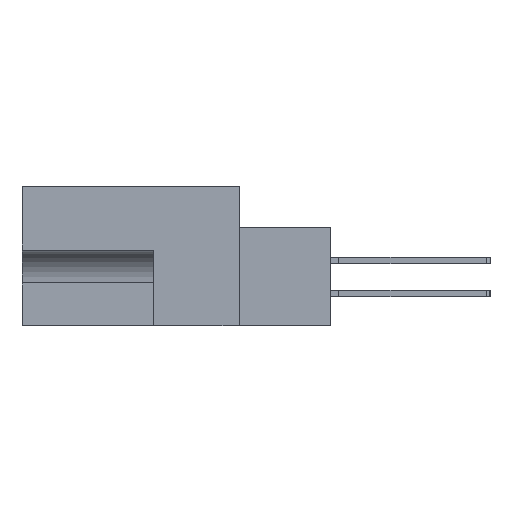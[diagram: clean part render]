
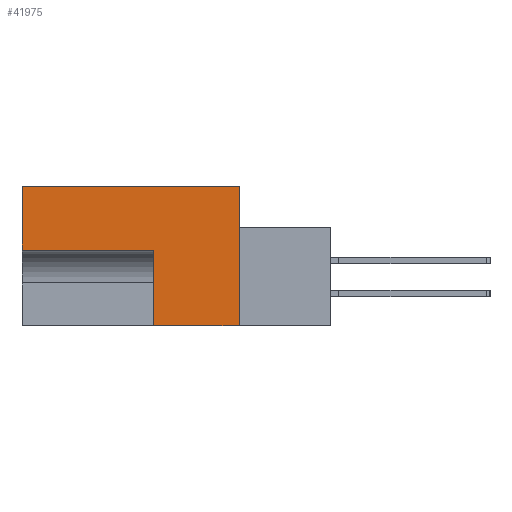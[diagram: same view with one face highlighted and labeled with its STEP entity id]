
A CAD part, left-side view. The second image highlights one B-rep face of the part: STEP entity #41975.
In plain terms, the highlighted planar face has unit normal (-1, 0, 0).
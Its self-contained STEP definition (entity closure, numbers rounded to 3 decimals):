
#271 = CARTESIAN_POINT ( 'NONE',  ( 0., 8.255, -6.172 ) ) ;
#619 = VERTEX_POINT ( 'NONE', #6439 ) ;
#1809 = EDGE_CURVE ( 'NONE', #14572, #31954, #23709, .T. ) ;
#2557 = VERTEX_POINT ( 'NONE', #12913 ) ;
#3191 = EDGE_CURVE ( 'NONE', #2557, #45416, #29184, .T. ) ;
#4300 = CARTESIAN_POINT ( 'NONE',  ( 0., -8.814, -13.487 ) ) ;
#6439 = CARTESIAN_POINT ( 'NONE',  ( 0., 8.255, -13.487 ) ) ;
#9288 = LINE ( 'NONE', #18768, #26078 ) ;
#10592 = VECTOR ( 'NONE', #28464, 1000. ) ;
#11209 = VERTEX_POINT ( 'NONE', #12838 ) ;
#11371 = VECTOR ( 'NONE', #39637, 1000. ) ;
#11710 = LINE ( 'NONE', #21311, #10592 ) ;
#12730 = CARTESIAN_POINT ( 'NONE',  ( 0., 8.255, -6.172 ) ) ;
#12799 = AXIS2_PLACEMENT_3D ( 'NONE', #17587, #14251, #21201 ) ;
#12838 = CARTESIAN_POINT ( 'NONE',  ( 0., 20.955, 0. ) ) ;
#12913 = CARTESIAN_POINT ( 'NONE',  ( 0., 0., 0. ) ) ;
#14251 = DIRECTION ( 'NONE',  ( 1., 0., 0. ) ) ;
#14572 = VERTEX_POINT ( 'NONE', #12730 ) ;
#16390 = DIRECTION ( 'NONE',  ( 0., 0., -1. ) ) ;
#17149 = VECTOR ( 'NONE', #31391, 1000. ) ;
#17314 = ORIENTED_EDGE ( 'NONE', *, *, #1809, .F. ) ;
#17430 = ORIENTED_EDGE ( 'NONE', *, *, #21284, .F. ) ;
#17587 = CARTESIAN_POINT ( 'NONE',  ( 0., 0., 0. ) ) ;
#18768 = CARTESIAN_POINT ( 'NONE',  ( 0., 11.506, 0. ) ) ;
#19644 = ORIENTED_EDGE ( 'NONE', *, *, #3191, .F. ) ;
#21201 = DIRECTION ( 'NONE',  ( 0., 0., -1. ) ) ;
#21284 = EDGE_CURVE ( 'NONE', #619, #14572, #11710, .T. ) ;
#21311 = CARTESIAN_POINT ( 'NONE',  ( 0., 8.255, -13.487 ) ) ;
#23709 = LINE ( 'NONE', #271, #11371 ) ;
#24546 = VECTOR ( 'NONE', #43676, 1000. ) ;
#24553 = EDGE_CURVE ( 'NONE', #11209, #2557, #9288, .T. ) ;
#24628 = PLANE ( 'NONE',  #12799 ) ;
#25852 = ORIENTED_EDGE ( 'NONE', *, *, #34204, .F. ) ;
#26078 = VECTOR ( 'NONE', #43744, 1000. ) ;
#27905 = EDGE_LOOP ( 'NONE', ( #38686, #19644, #41209, #25852, #17314, #17430 ) ) ;
#28117 = CARTESIAN_POINT ( 'NONE',  ( 0., 20.955, -13.487 ) ) ;
#28464 = DIRECTION ( 'NONE',  ( 0., 0., 1. ) ) ;
#29184 = LINE ( 'NONE', #37662, #32545 ) ;
#30675 = LINE ( 'NONE', #4300, #24546 ) ;
#31391 = DIRECTION ( 'NONE',  ( 0., 0., 1. ) ) ;
#31954 = VERTEX_POINT ( 'NONE', #38994 ) ;
#32545 = VECTOR ( 'NONE', #16390, 1000. ) ;
#34204 = EDGE_CURVE ( 'NONE', #31954, #11209, #45642, .T. ) ;
#37662 = CARTESIAN_POINT ( 'NONE',  ( 0., 0., 0. ) ) ;
#38686 = ORIENTED_EDGE ( 'NONE', *, *, #40483, .F. ) ;
#38994 = CARTESIAN_POINT ( 'NONE',  ( 0., 20.955, -6.172 ) ) ;
#39637 = DIRECTION ( 'NONE',  ( 0., 1., 0. ) ) ;
#40483 = EDGE_CURVE ( 'NONE', #45416, #619, #30675, .T. ) ;
#41209 = ORIENTED_EDGE ( 'NONE', *, *, #24553, .F. ) ;
#41975 = ADVANCED_FACE ( 'NONE', ( #45611 ), #24628, .F. ) ;
#43676 = DIRECTION ( 'NONE',  ( 0., 1., 0. ) ) ;
#43744 = DIRECTION ( 'NONE',  ( 0., -1., 0. ) ) ;
#44670 = CARTESIAN_POINT ( 'NONE',  ( 0., 0., -13.487 ) ) ;
#45416 = VERTEX_POINT ( 'NONE', #44670 ) ;
#45611 = FACE_OUTER_BOUND ( 'NONE', #27905, .T. ) ;
#45642 = LINE ( 'NONE', #28117, #17149 ) ;
